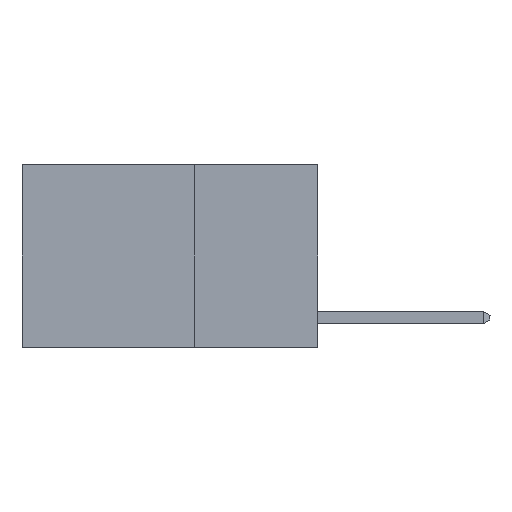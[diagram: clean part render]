
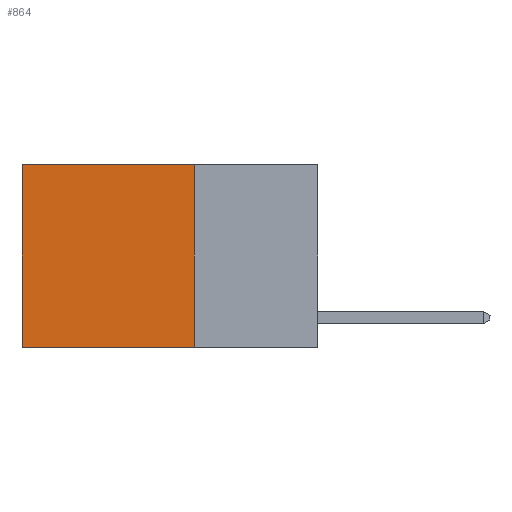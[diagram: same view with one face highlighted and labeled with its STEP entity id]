
A CAD part, left-side view. The second image highlights one B-rep face of the part: STEP entity #864.
In plain terms, the highlighted planar face has unit normal (-1, 0, 0).
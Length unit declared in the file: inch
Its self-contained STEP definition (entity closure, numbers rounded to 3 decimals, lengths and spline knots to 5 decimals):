
#123 = EDGE_CURVE ( 'NONE', #9803, #7915, #3972, .T. ) ;
#451 = CARTESIAN_POINT ( 'NONE',  ( 0.2625, 0.25, 0. ) ) ;
#481 = EDGE_CURVE ( 'NONE', #10230, #9803, #1725, .T. ) ;
#534 = DIRECTION ( 'NONE',  ( 0., 1., 0. ) ) ;
#613 = ORIENTED_EDGE ( 'NONE', *, *, #123, .F. ) ;
#860 = ORIENTED_EDGE ( 'NONE', *, *, #3666, .T. ) ;
#864 = ADVANCED_FACE ( 'NONE', ( #6460 ), #8859, .F. ) ;
#868 = ORIENTED_EDGE ( 'NONE', *, *, #481, .F. ) ;
#898 = CARTESIAN_POINT ( 'NONE',  ( 0.2625, 0.25, 0. ) ) ;
#1725 = LINE ( 'NONE', #5754, #10351 ) ;
#2358 = DIRECTION ( 'NONE',  ( 0., 1., 0. ) ) ;
#3301 = CARTESIAN_POINT ( 'NONE',  ( 0.2625, 0.25, -0.37 ) ) ;
#3425 = AXIS2_PLACEMENT_3D ( 'NONE', #898, #9727, #4145 ) ;
#3666 = EDGE_CURVE ( 'NONE', #10230, #8479, #4542, .T. ) ;
#3826 = EDGE_CURVE ( 'NONE', #8479, #7915, #9467, .T. ) ;
#3972 = LINE ( 'NONE', #7752, #6242 ) ;
#4145 = DIRECTION ( 'NONE',  ( 0., 0., -1. ) ) ;
#4542 = LINE ( 'NONE', #451, #6063 ) ;
#5124 = ORIENTED_EDGE ( 'NONE', *, *, #3826, .T. ) ;
#5734 = VECTOR ( 'NONE', #6264, 39.37008 ) ;
#5754 = CARTESIAN_POINT ( 'NONE',  ( 0.2625, 0.25, 0. ) ) ;
#6063 = VECTOR ( 'NONE', #2358, 39.37008 ) ;
#6242 = VECTOR ( 'NONE', #534, 39.37008 ) ;
#6264 = DIRECTION ( 'NONE',  ( 0., 0., -1. ) ) ;
#6309 = CARTESIAN_POINT ( 'NONE',  ( 0.2625, 0.6, 0. ) ) ;
#6460 = FACE_OUTER_BOUND ( 'NONE', #10272, .T. ) ;
#7189 = CARTESIAN_POINT ( 'NONE',  ( 0.2625, 0.6, -0.37 ) ) ;
#7752 = CARTESIAN_POINT ( 'NONE',  ( 0.2625, 0.25, -0.37 ) ) ;
#7915 = VERTEX_POINT ( 'NONE', #7189 ) ;
#8192 = DIRECTION ( 'NONE',  ( 0., 0., -1. ) ) ;
#8479 = VERTEX_POINT ( 'NONE', #9453 ) ;
#8620 = CARTESIAN_POINT ( 'NONE',  ( 0.2625, 0.25, 0. ) ) ;
#8859 = PLANE ( 'NONE',  #3425 ) ;
#9453 = CARTESIAN_POINT ( 'NONE',  ( 0.2625, 0.6, 0. ) ) ;
#9467 = LINE ( 'NONE', #6309, #5734 ) ;
#9727 = DIRECTION ( 'NONE',  ( 1., 0., 0. ) ) ;
#9803 = VERTEX_POINT ( 'NONE', #3301 ) ;
#10230 = VERTEX_POINT ( 'NONE', #8620 ) ;
#10272 = EDGE_LOOP ( 'NONE', ( #5124, #613, #868, #860 ) ) ;
#10351 = VECTOR ( 'NONE', #8192, 39.37008 ) ;
